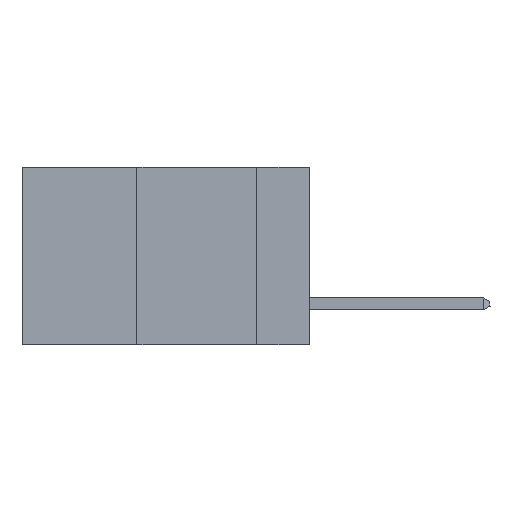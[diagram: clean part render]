
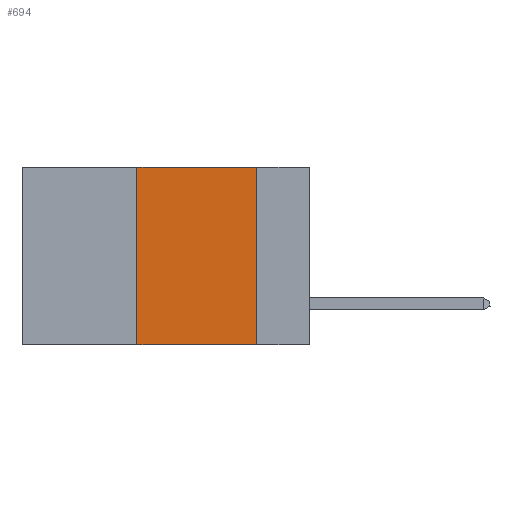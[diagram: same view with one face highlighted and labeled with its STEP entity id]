
A CAD part, left-side view. The second image highlights one B-rep face of the part: STEP entity #694.
In plain terms, the highlighted planar face has unit normal (-1, 0, 0).
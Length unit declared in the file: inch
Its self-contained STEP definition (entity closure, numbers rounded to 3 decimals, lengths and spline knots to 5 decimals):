
#694 = ADVANCED_FACE ( 'NONE', ( #1315 ), #8083, .F. ) ;
#809 = DIRECTION ( 'NONE',  ( 0., 0., 1. ) ) ;
#876 = CARTESIAN_POINT ( 'NONE',  ( 0., 0.36, 0. ) ) ;
#1315 = FACE_OUTER_BOUND ( 'NONE', #9987, .T. ) ;
#1562 = EDGE_CURVE ( 'NONE', #5325, #2063, #5781, .T. ) ;
#1712 = LINE ( 'NONE', #14525, #7230 ) ;
#1874 = CARTESIAN_POINT ( 'NONE',  ( 0., 0.6, 0. ) ) ;
#1955 = VERTEX_POINT ( 'NONE', #7037 ) ;
#2063 = VERTEX_POINT ( 'NONE', #13691 ) ;
#3542 = LINE ( 'NONE', #3749, #4033 ) ;
#3749 = CARTESIAN_POINT ( 'NONE',  ( 0., 0.36, 0. ) ) ;
#4033 = VECTOR ( 'NONE', #809, 39.37008 ) ;
#5225 = ORIENTED_EDGE ( 'NONE', *, *, #19353, .T. ) ;
#5325 = VERTEX_POINT ( 'NONE', #8241 ) ;
#5781 = LINE ( 'NONE', #7250, #19909 ) ;
#7037 = CARTESIAN_POINT ( 'NONE',  ( 0., 0.36, -0.37 ) ) ;
#7230 = VECTOR ( 'NONE', #14596, 39.37008 ) ;
#7250 = CARTESIAN_POINT ( 'NONE',  ( 0., 0.11, 0. ) ) ;
#7356 = ORIENTED_EDGE ( 'NONE', *, *, #1562, .F. ) ;
#7681 = AXIS2_PLACEMENT_3D ( 'NONE', #1874, #13022, #13092 ) ;
#8083 = PLANE ( 'NONE',  #7681 ) ;
#8241 = CARTESIAN_POINT ( 'NONE',  ( 0., 0.11, 0. ) ) ;
#9218 = VECTOR ( 'NONE', #13840, 39.37008 ) ;
#9987 = EDGE_LOOP ( 'NONE', ( #7356, #17354, #14059, #5225 ) ) ;
#11215 = LINE ( 'NONE', #18474, #9218 ) ;
#12485 = EDGE_CURVE ( 'NONE', #1955, #12688, #3542, .T. ) ;
#12688 = VERTEX_POINT ( 'NONE', #876 ) ;
#13022 = DIRECTION ( 'NONE',  ( 1., 0., 0. ) ) ;
#13092 = DIRECTION ( 'NONE',  ( 0., 0., -1. ) ) ;
#13691 = CARTESIAN_POINT ( 'NONE',  ( 0., 0.11, -0.37 ) ) ;
#13840 = DIRECTION ( 'NONE',  ( 0., -1., 0. ) ) ;
#14059 = ORIENTED_EDGE ( 'NONE', *, *, #12485, .F. ) ;
#14525 = CARTESIAN_POINT ( 'NONE',  ( 0., 0.6, -0.37 ) ) ;
#14596 = DIRECTION ( 'NONE',  ( 0., -1., 0. ) ) ;
#17354 = ORIENTED_EDGE ( 'NONE', *, *, #18460, .F. ) ;
#18460 = EDGE_CURVE ( 'NONE', #12688, #5325, #11215, .T. ) ;
#18474 = CARTESIAN_POINT ( 'NONE',  ( 0., 0.6, 0. ) ) ;
#18543 = DIRECTION ( 'NONE',  ( 0., 0., -1. ) ) ;
#19353 = EDGE_CURVE ( 'NONE', #1955, #2063, #1712, .T. ) ;
#19909 = VECTOR ( 'NONE', #18543, 39.37008 ) ;
